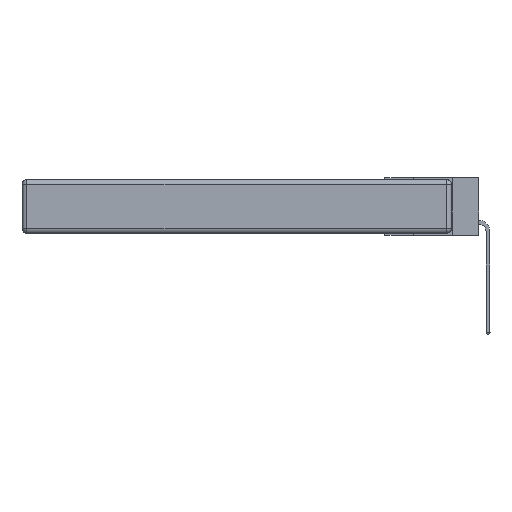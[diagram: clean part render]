
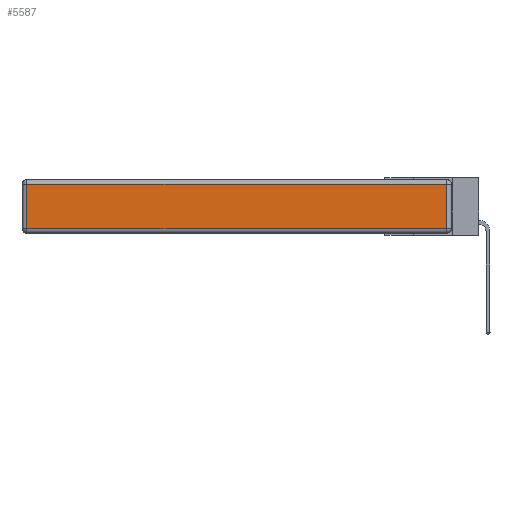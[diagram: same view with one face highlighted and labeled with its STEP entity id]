
A CAD part, left-side view. The second image highlights one B-rep face of the part: STEP entity #5587.
In plain terms, the highlighted planar face has unit normal (-1, 0, 0).
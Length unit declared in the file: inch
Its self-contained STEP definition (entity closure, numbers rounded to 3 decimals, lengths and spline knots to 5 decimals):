
#750 = AXIS2_PLACEMENT_3D ( 'NONE', #1957, #20972, #13798 ) ;
#1830 = EDGE_CURVE ( 'NONE', #8519, #28094, #22080, .T. ) ;
#1957 = CARTESIAN_POINT ( 'NONE',  ( 0., 0., -0.343 ) ) ;
#3594 = LINE ( 'NONE', #23578, #23476 ) ;
#4510 = ORIENTED_EDGE ( 'NONE', *, *, #18356, .T. ) ;
#5587 = ADVANCED_FACE ( 'NONE', ( #30407 ), #8774, .T. ) ;
#5932 = DIRECTION ( 'NONE',  ( 0., 0., 1. ) ) ;
#6021 = CARTESIAN_POINT ( 'NONE',  ( 0., 0.03, -0.343 ) ) ;
#6286 = VECTOR ( 'NONE', #5932, 39.37008 ) ;
#8154 = EDGE_LOOP ( 'NONE', ( #18083, #30323, #22936, #4510 ) ) ;
#8519 = VERTEX_POINT ( 'NONE', #29027 ) ;
#8774 = PLANE ( 'NONE',  #750 ) ;
#10552 = EDGE_CURVE ( 'NONE', #28094, #13740, #16758, .T. ) ;
#10826 = EDGE_CURVE ( 'NONE', #24551, #8519, #15597, .T. ) ;
#13557 = CARTESIAN_POINT ( 'NONE',  ( 0., 2.72, -0.313 ) ) ;
#13740 = VERTEX_POINT ( 'NONE', #15896 ) ;
#13798 = DIRECTION ( 'NONE',  ( 0., 0., 1. ) ) ;
#15051 = CARTESIAN_POINT ( 'NONE',  ( 0., 2.75, -0.03 ) ) ;
#15467 = DIRECTION ( 'NONE',  ( 0., 1., 0. ) ) ;
#15597 = LINE ( 'NONE', #20809, #19018 ) ;
#15896 = CARTESIAN_POINT ( 'NONE',  ( 0., 2.72, -0.03 ) ) ;
#16758 = LINE ( 'NONE', #15051, #20935 ) ;
#18083 = ORIENTED_EDGE ( 'NONE', *, *, #10826, .T. ) ;
#18356 = EDGE_CURVE ( 'NONE', #13740, #24551, #3594, .T. ) ;
#19018 = VECTOR ( 'NONE', #30087, 39.37008 ) ;
#20809 = CARTESIAN_POINT ( 'NONE',  ( 0., 0., -0.313 ) ) ;
#20819 = CARTESIAN_POINT ( 'NONE',  ( 0., 0.03, -0.03 ) ) ;
#20935 = VECTOR ( 'NONE', #15467, 39.37008 ) ;
#20972 = DIRECTION ( 'NONE',  ( -1., 0., 0. ) ) ;
#22080 = LINE ( 'NONE', #6021, #6286 ) ;
#22936 = ORIENTED_EDGE ( 'NONE', *, *, #10552, .T. ) ;
#23467 = DIRECTION ( 'NONE',  ( 0., 0., -1. ) ) ;
#23476 = VECTOR ( 'NONE', #23467, 39.37008 ) ;
#23578 = CARTESIAN_POINT ( 'NONE',  ( 0., 2.72, -0.343 ) ) ;
#24551 = VERTEX_POINT ( 'NONE', #13557 ) ;
#28094 = VERTEX_POINT ( 'NONE', #20819 ) ;
#29027 = CARTESIAN_POINT ( 'NONE',  ( 0., 0.03, -0.313 ) ) ;
#30087 = DIRECTION ( 'NONE',  ( 0., -1., 0. ) ) ;
#30323 = ORIENTED_EDGE ( 'NONE', *, *, #1830, .T. ) ;
#30407 = FACE_OUTER_BOUND ( 'NONE', #8154, .T. ) ;
